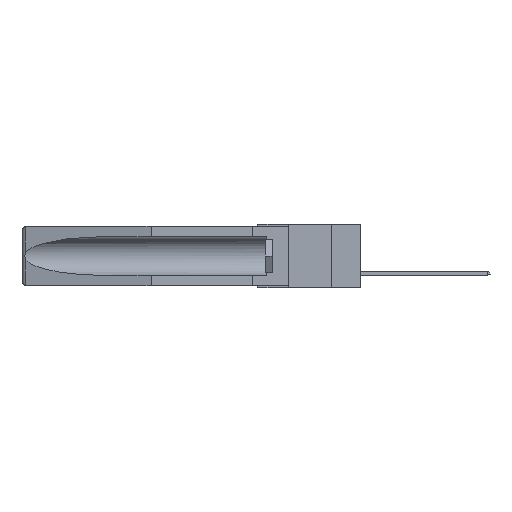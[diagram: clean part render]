
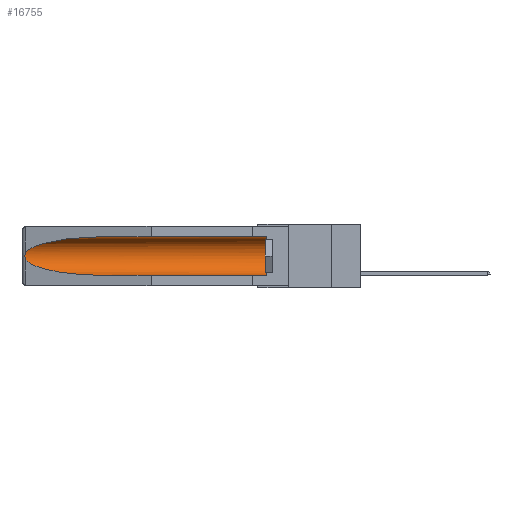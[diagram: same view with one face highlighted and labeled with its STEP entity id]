
A CAD part, left-side view. The second image highlights one B-rep face of the part: STEP entity #16755.
In plain terms, the highlighted cylindrical face has radius 2.857 mm (diameter 5.715 mm), a partial arc.
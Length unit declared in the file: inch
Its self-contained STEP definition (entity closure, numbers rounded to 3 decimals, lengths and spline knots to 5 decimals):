
#149 = DIRECTION ( 'NONE',  ( 0., 1., 0. ) ) ;
#521 = CARTESIAN_POINT ( 'NONE',  ( 0.155, 1.07973, -0.284 ) ) ;
#1157 = CARTESIAN_POINT ( 'NONE',  ( 0.26537, 1.52718, -0.14972 ) ) ;
#1871 = EDGE_CURVE ( 'NONE', #17059, #8359, #21895, .T. ) ;
#1959 = VECTOR ( 'NONE', #149, 39.37008 ) ;
#2524 = CARTESIAN_POINT ( 'NONE',  ( 0.155, 1.07973, -0.059 ) ) ;
#2657 = CARTESIAN_POINT ( 'NONE',  ( 0.25451, 1.48313, -0.09465 ) ) ;
#3290 = DIRECTION ( 'NONE',  ( 0., 1., 0. ) ) ;
#3731 = EDGE_CURVE ( 'NONE', #7640, #14023, #18424, .T. ) ;
#4542 = CARTESIAN_POINT ( 'NONE',  ( 0.155, 0.126, -0.059 ) ) ;
#5860 = CARTESIAN_POINT ( 'NONE',  ( 0.2673, 1.53269, -0.17917 ) ) ;
#5897 = CARTESIAN_POINT ( 'NONE',  ( 0.155, 0.126, -0.1715 ) ) ;
#5941 = CARTESIAN_POINT ( 'NONE',  ( 0.155, 1.07973, -0.059 ) ) ;
#6088 = CARTESIAN_POINT ( 'NONE',  ( 0.2673, 1.5327, -0.16383 ) ) ;
#6247 = CARTESIAN_POINT ( 'NONE',  ( 0.25451, 1.48313, -0.24835 ) ) ;
#6266 = ORIENTED_EDGE ( 'NONE', *, *, #3731, .T. ) ;
#6388 = EDGE_CURVE ( 'NONE', #20721, #7640, #8409, .T. ) ;
#6653 = EDGE_CURVE ( 'NONE', #17059, #8866, #20069, .T. ) ;
#7573 = CARTESIAN_POINT ( 'NONE',  ( 0.26597, 1.5296, -0.19026 ) ) ;
#7640 = VERTEX_POINT ( 'NONE', #1157 ) ;
#7653 = CARTESIAN_POINT ( 'NONE',  ( 0.2675, 1.53308, -0.16763 ) ) ;
#8359 = VERTEX_POINT ( 'NONE', #4542 ) ;
#8409 =( BOUNDED_CURVE ( )  B_SPLINE_CURVE ( 3, ( #5941, #21333, #2657, #17828 ),
 .UNSPECIFIED., .F., .F. ) 
 B_SPLINE_CURVE_WITH_KNOTS ( ( 4, 4 ),
 ( 4.71239, 6.08839 ),
 .UNSPECIFIED. ) 
 CURVE ( )  GEOMETRIC_REPRESENTATION_ITEM ( )  RATIONAL_B_SPLINE_CURVE ( ( 1., 0.848, 0.848, 1. ) ) 
 REPRESENTATION_ITEM ( '' )  );
#8457 = DIRECTION ( 'NONE',  ( 0., 1., 0. ) ) ;
#8804 = CARTESIAN_POINT ( 'NONE',  ( 0.155, -0.30754, -0.059 ) ) ;
#8866 = VERTEX_POINT ( 'NONE', #521 ) ;
#8893 = LINE ( 'NONE', #8804, #1959 ) ;
#9076 =( BOUNDED_CURVE ( )  B_SPLINE_CURVE ( 3, ( #16503, #6247, #19918, #9675 ),
 .UNSPECIFIED., .F., .F. ) 
 B_SPLINE_CURVE_WITH_KNOTS ( ( 4, 4 ),
 ( 0.1948, 1.5708 ),
 .UNSPECIFIED. ) 
 CURVE ( )  GEOMETRIC_REPRESENTATION_ITEM ( )  RATIONAL_B_SPLINE_CURVE ( ( 1., 0.848, 0.848, 1. ) ) 
 REPRESENTATION_ITEM ( '' )  );
#9177 = AXIS2_PLACEMENT_3D ( 'NONE', #5897, #16232, #10921 ) ;
#9442 = CARTESIAN_POINT ( 'NONE',  ( 0.26654, 1.53092, -0.15636 ) ) ;
#9518 = CARTESIAN_POINT ( 'NONE',  ( 0.26537, 1.52718, -0.14972 ) ) ;
#9675 = CARTESIAN_POINT ( 'NONE',  ( 0.155, 1.07973, -0.284 ) ) ;
#9780 = EDGE_CURVE ( 'NONE', #14023, #8866, #9076, .T. ) ;
#9788 = FACE_OUTER_BOUND ( 'NONE', #20031, .T. ) ;
#10883 = ORIENTED_EDGE ( 'NONE', *, *, #1871, .T. ) ;
#10921 = DIRECTION ( 'NONE',  ( 0., 0., 1. ) ) ;
#12063 = EDGE_CURVE ( 'NONE', #8359, #20721, #8893, .T. ) ;
#12248 = ORIENTED_EDGE ( 'NONE', *, *, #6653, .F. ) ;
#12815 = ORIENTED_EDGE ( 'NONE', *, *, #6388, .T. ) ;
#12879 = CARTESIAN_POINT ( 'NONE',  ( 0.26655, 1.53094, -0.18657 ) ) ;
#13350 = CARTESIAN_POINT ( 'NONE',  ( 0.155, -0.30754, -0.1715 ) ) ;
#13565 = DIRECTION ( 'NONE',  ( 0., 0., 1. ) ) ;
#14023 = VERTEX_POINT ( 'NONE', #16251 ) ;
#14233 = CARTESIAN_POINT ( 'NONE',  ( 0.155, 0.126, -0.284 ) ) ;
#14420 = CARTESIAN_POINT ( 'NONE',  ( 0.2675, 1.53308, -0.17534 ) ) ;
#14483 = VECTOR ( 'NONE', #3290, 39.37008 ) ;
#14773 = ORIENTED_EDGE ( 'NONE', *, *, #12063, .T. ) ;
#16232 = DIRECTION ( 'NONE',  ( 0., -1., 0. ) ) ;
#16251 = CARTESIAN_POINT ( 'NONE',  ( 0.26537, 1.52718, -0.19328 ) ) ;
#16269 = CARTESIAN_POINT ( 'NONE',  ( 0.26597, 1.52961, -0.15275 ) ) ;
#16503 = CARTESIAN_POINT ( 'NONE',  ( 0.26537, 1.52718, -0.19328 ) ) ;
#16624 = ORIENTED_EDGE ( 'NONE', *, *, #9780, .T. ) ;
#16755 = ADVANCED_FACE ( 'NONE', ( #9788 ), #18638, .F. ) ;
#17059 = VERTEX_POINT ( 'NONE', #14233 ) ;
#17828 = CARTESIAN_POINT ( 'NONE',  ( 0.26537, 1.52718, -0.14972 ) ) ;
#18424 = B_SPLINE_CURVE_WITH_KNOTS ( 'NONE', 3,
 ( #9518, #16269, #9442, #6088, #7653, #14420, #5860, #12879, #7573, #19465 ),
 .UNSPECIFIED., .F., .F.,
 ( 4, 2, 2, 2, 4 ),
 ( 0., 0.00029, 0.00058, 0.00087, 0.00117 ),
 .UNSPECIFIED. ) ;
#18638 = CYLINDRICAL_SURFACE ( 'NONE', #20571, 0.1125 ) ;
#19465 = CARTESIAN_POINT ( 'NONE',  ( 0.26537, 1.52718, -0.19328 ) ) ;
#19918 = CARTESIAN_POINT ( 'NONE',  ( 0.21114, 1.30732, -0.284 ) ) ;
#20031 = EDGE_LOOP ( 'NONE', ( #12815, #6266, #16624, #12248, #10883, #14773 ) ) ;
#20069 = LINE ( 'NONE', #20216, #14483 ) ;
#20216 = CARTESIAN_POINT ( 'NONE',  ( 0.155, -0.30754, -0.284 ) ) ;
#20571 = AXIS2_PLACEMENT_3D ( 'NONE', #13350, #8457, #13565 ) ;
#20721 = VERTEX_POINT ( 'NONE', #2524 ) ;
#21333 = CARTESIAN_POINT ( 'NONE',  ( 0.21114, 1.30732, -0.059 ) ) ;
#21895 = CIRCLE ( 'NONE', #9177, 0.1125 ) ;
